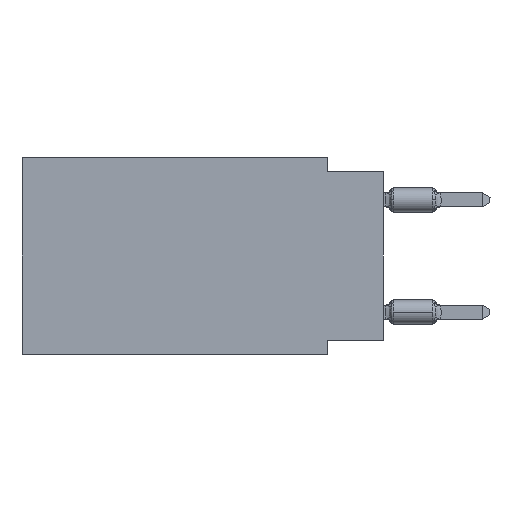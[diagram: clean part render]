
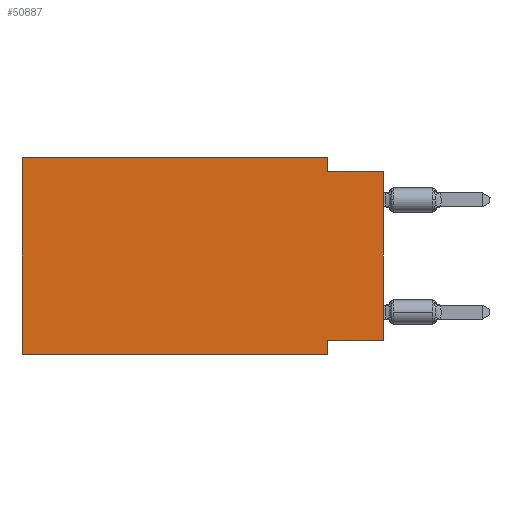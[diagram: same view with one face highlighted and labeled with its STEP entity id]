
A CAD part, left-side view. The second image highlights one B-rep face of the part: STEP entity #50887.
In plain terms, the highlighted planar face has unit normal (-1, 0, 0).
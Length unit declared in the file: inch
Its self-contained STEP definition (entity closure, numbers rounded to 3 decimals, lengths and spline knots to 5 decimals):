
#277 = EDGE_CURVE ( 'NONE', #15087, #51564, #43555, .T. ) ;
#418 = CARTESIAN_POINT ( 'NONE',  ( 0., 0.645, 0. ) ) ;
#439 = VERTEX_POINT ( 'NONE', #34138 ) ;
#849 = LINE ( 'NONE', #25550, #5581 ) ;
#1714 = LINE ( 'NONE', #21548, #47040 ) ;
#2903 = ORIENTED_EDGE ( 'NONE', *, *, #59451, .F. ) ;
#3928 = DIRECTION ( 'NONE',  ( 0., -1., 0. ) ) ;
#4450 = ORIENTED_EDGE ( 'NONE', *, *, #277, .F. ) ;
#5581 = VECTOR ( 'NONE', #11856, 39.37008 ) ;
#6212 = CARTESIAN_POINT ( 'NONE',  ( 0., 0.1, -0.35 ) ) ;
#6960 = ORIENTED_EDGE ( 'NONE', *, *, #10738, .T. ) ;
#7931 = VERTEX_POINT ( 'NONE', #24718 ) ;
#9655 = FACE_OUTER_BOUND ( 'NONE', #36131, .T. ) ;
#10067 = VECTOR ( 'NONE', #3928, 39.37008 ) ;
#10738 = EDGE_CURVE ( 'NONE', #439, #7931, #20431, .T. ) ;
#11856 = DIRECTION ( 'NONE',  ( 0., 0., 1. ) ) ;
#12068 = VECTOR ( 'NONE', #60944, 39.37008 ) ;
#14957 = VERTEX_POINT ( 'NONE', #44078 ) ;
#15087 = VERTEX_POINT ( 'NONE', #34980 ) ;
#20431 = LINE ( 'NONE', #30460, #57599 ) ;
#21548 = CARTESIAN_POINT ( 'NONE',  ( 0., 0., -0.325 ) ) ;
#21611 = CARTESIAN_POINT ( 'NONE',  ( 0., 0.1, 0. ) ) ;
#22457 = DIRECTION ( 'NONE',  ( 0., 0., -1. ) ) ;
#23291 = EDGE_CURVE ( 'NONE', #14957, #62399, #849, .T. ) ;
#23403 = CARTESIAN_POINT ( 'NONE',  ( 0., 0., -0.025 ) ) ;
#23416 = CARTESIAN_POINT ( 'NONE',  ( 0., 0.1, -0.35 ) ) ;
#23801 = VECTOR ( 'NONE', #61207, 39.37008 ) ;
#24718 = CARTESIAN_POINT ( 'NONE',  ( 0., 0., -0.025 ) ) ;
#25096 = ORIENTED_EDGE ( 'NONE', *, *, #59803, .F. ) ;
#25459 = ORIENTED_EDGE ( 'NONE', *, *, #48118, .F. ) ;
#25550 = CARTESIAN_POINT ( 'NONE',  ( 0., 0.645, 0. ) ) ;
#29497 = DIRECTION ( 'NONE',  ( 0., 0., -1. ) ) ;
#30460 = CARTESIAN_POINT ( 'NONE',  ( 0., 0., 0. ) ) ;
#30732 = EDGE_CURVE ( 'NONE', #63208, #57142, #31026, .T. ) ;
#31026 = LINE ( 'NONE', #21611, #23801 ) ;
#33387 = PLANE ( 'NONE',  #34611 ) ;
#34138 = CARTESIAN_POINT ( 'NONE',  ( 0., 0., -0.325 ) ) ;
#34232 = DIRECTION ( 'NONE',  ( 0., -1., 0. ) ) ;
#34500 = CARTESIAN_POINT ( 'NONE',  ( 0., 0.1, 0. ) ) ;
#34611 = AXIS2_PLACEMENT_3D ( 'NONE', #53193, #38577, #29497 ) ;
#34980 = CARTESIAN_POINT ( 'NONE',  ( 0., 0.1, -0.325 ) ) ;
#35946 = LINE ( 'NONE', #41159, #12068 ) ;
#36131 = EDGE_LOOP ( 'NONE', ( #6960, #25459, #57536, #25096, #63165, #42987, #4450, #2903 ) ) ;
#38577 = DIRECTION ( 'NONE',  ( 1., 0., 0. ) ) ;
#39142 = CARTESIAN_POINT ( 'NONE',  ( 0., 0.1, -0.025 ) ) ;
#41086 = DIRECTION ( 'NONE',  ( 0., 1., 0. ) ) ;
#41159 = CARTESIAN_POINT ( 'NONE',  ( 0., 0.645, -0.35 ) ) ;
#42163 = EDGE_CURVE ( 'NONE', #14957, #51564, #35946, .T. ) ;
#42987 = ORIENTED_EDGE ( 'NONE', *, *, #42163, .T. ) ;
#43555 = LINE ( 'NONE', #23416, #44725 ) ;
#43833 = CARTESIAN_POINT ( 'NONE',  ( 0., 0.645, 0. ) ) ;
#44078 = CARTESIAN_POINT ( 'NONE',  ( 0., 0.645, -0.35 ) ) ;
#44725 = VECTOR ( 'NONE', #22457, 39.37008 ) ;
#47040 = VECTOR ( 'NONE', #41086, 39.37008 ) ;
#48118 = EDGE_CURVE ( 'NONE', #57142, #7931, #52644, .T. ) ;
#50117 = LINE ( 'NONE', #418, #56359 ) ;
#50294 = DIRECTION ( 'NONE',  ( 0., 0., 1. ) ) ;
#50887 = ADVANCED_FACE ( 'NONE', ( #9655 ), #33387, .F. ) ;
#51564 = VERTEX_POINT ( 'NONE', #6212 ) ;
#52644 = LINE ( 'NONE', #23403, #10067 ) ;
#53193 = CARTESIAN_POINT ( 'NONE',  ( 0., 0.645, 0. ) ) ;
#56359 = VECTOR ( 'NONE', #34232, 39.37008 ) ;
#57142 = VERTEX_POINT ( 'NONE', #39142 ) ;
#57536 = ORIENTED_EDGE ( 'NONE', *, *, #30732, .F. ) ;
#57599 = VECTOR ( 'NONE', #50294, 39.37008 ) ;
#59451 = EDGE_CURVE ( 'NONE', #439, #15087, #1714, .T. ) ;
#59803 = EDGE_CURVE ( 'NONE', #62399, #63208, #50117, .T. ) ;
#60944 = DIRECTION ( 'NONE',  ( 0., -1., 0. ) ) ;
#61207 = DIRECTION ( 'NONE',  ( 0., 0., -1. ) ) ;
#62399 = VERTEX_POINT ( 'NONE', #43833 ) ;
#63165 = ORIENTED_EDGE ( 'NONE', *, *, #23291, .F. ) ;
#63208 = VERTEX_POINT ( 'NONE', #34500 ) ;
